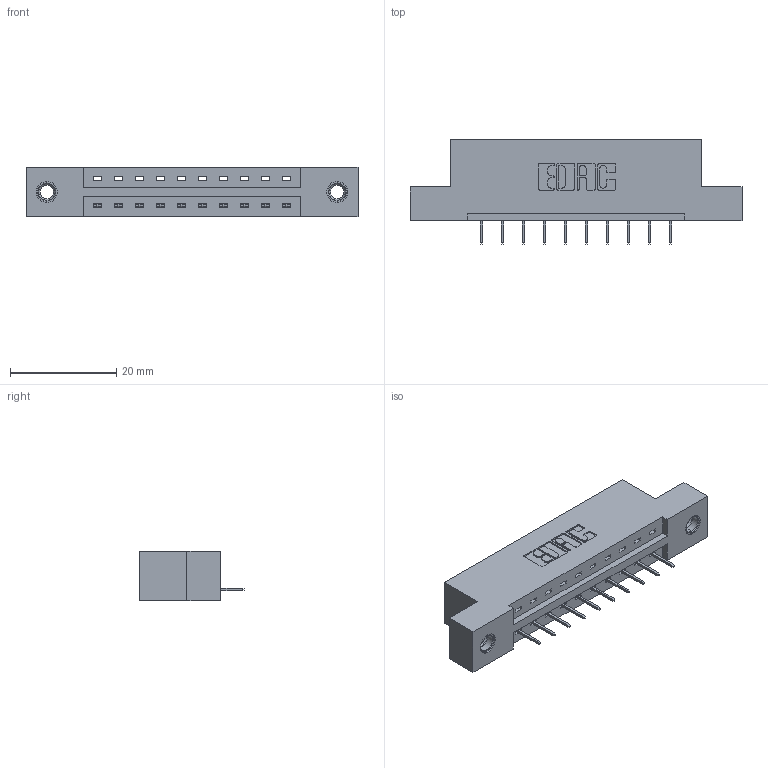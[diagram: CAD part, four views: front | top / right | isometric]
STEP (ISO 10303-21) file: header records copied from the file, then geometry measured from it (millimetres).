
FILE_DESCRIPTION (( 'STEP AP203' ), '1' );
FILE_NAME ('387-010-524-107.STEP', '2019-10-02T11:16:03', ( '' ), ( '' ), 'SwSTEP 2.0', 'SolidWorks 2016', '' );
FILE_SCHEMA (( 'CONFIG_CONTROL_DESIGN' ));
Length unit declared in the file: inch
Products named in the file (4): 387-010-524-107; 345-292-001_345-293-124; 345-250-001_345-250-005-103; 337 Part_Flush Mounting Lugs - 0.156 Dia-TI
Assembly tree (13 placements, depth 2):
  387-010-524-107
    337 Part_Flush Mounting Lugs - 0.156 Dia-TI
    345-292-001_345-293-124  x10
    345-250-001_345-250-005-103  x2
Bounding box: 62.64 x 19.69 x 9.4 mm (x, y, z)
Volume: 6056.5 mm3; surface area: 5983.1 mm2
Topology: 13 solids, 13 shells, 834 faces, 2367 edges, 1530 vertices
Faces by surface type: plane 622, cylinder 196, cone 12, torus 4
Entity records: 12832 total; most frequent: CARTESIAN_POINT 2211, ORIENTED_EDGE 2150, DIRECTION 1961, EDGE_CURVE 1075, LINE 931, VECTOR 931, VERTEX_POINT 708, AXIS2_PLACEMENT_3D 515
